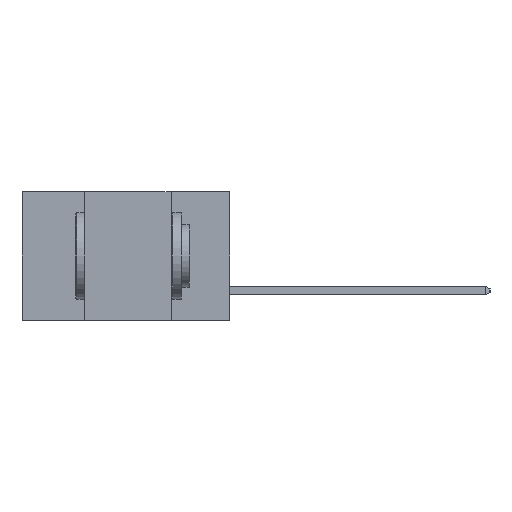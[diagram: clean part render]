
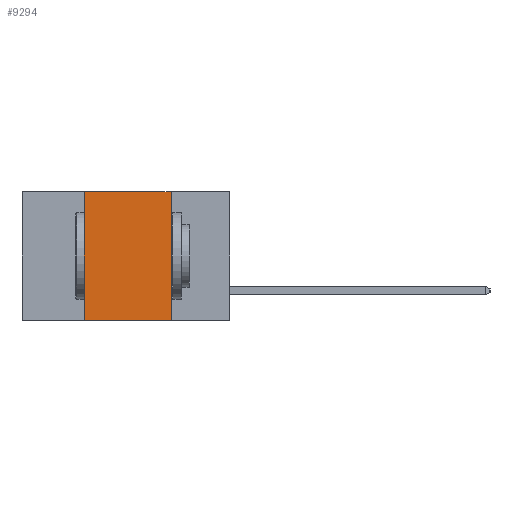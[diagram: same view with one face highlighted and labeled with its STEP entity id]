
A CAD part, left-side view. The second image highlights one B-rep face of the part: STEP entity #9294.
In plain terms, the highlighted planar face has unit normal (-1, 0, 0).
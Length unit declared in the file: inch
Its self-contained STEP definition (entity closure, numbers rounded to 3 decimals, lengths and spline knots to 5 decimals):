
#450 = ORIENTED_EDGE ( 'NONE', *, *, #6296, .F. ) ;
#673 = DIRECTION ( 'NONE',  ( 0., -1., 0. ) ) ;
#678 = LINE ( 'NONE', #5184, #2818 ) ;
#725 = DIRECTION ( 'NONE',  ( 0., -1., 0. ) ) ;
#744 = CARTESIAN_POINT ( 'NONE',  ( 0., 0.6, 0. ) ) ;
#784 = VECTOR ( 'NONE', #1436, 39.37008 ) ;
#842 = EDGE_CURVE ( 'NONE', #9845, #8155, #5381, .T. ) ;
#1018 = LINE ( 'NONE', #9768, #9151 ) ;
#1237 = EDGE_CURVE ( 'NONE', #9845, #6654, #1018, .T. ) ;
#1336 = ORIENTED_EDGE ( 'NONE', *, *, #1237, .T. ) ;
#1436 = DIRECTION ( 'NONE',  ( 0., 0., 1. ) ) ;
#1441 = CARTESIAN_POINT ( 'NONE',  ( 0., 0.42, -0.37 ) ) ;
#1471 = DIRECTION ( 'NONE',  ( 0., 0., -1. ) ) ;
#2467 = EDGE_CURVE ( 'NONE', #8155, #4888, #8090, .T. ) ;
#2547 = CARTESIAN_POINT ( 'NONE',  ( 0., 0.42, 0. ) ) ;
#2800 = CARTESIAN_POINT ( 'NONE',  ( 0., 0.17, -0.37 ) ) ;
#2818 = VECTOR ( 'NONE', #5220, 39.37008 ) ;
#2883 = ORIENTED_EDGE ( 'NONE', *, *, #2467, .F. ) ;
#2986 = ORIENTED_EDGE ( 'NONE', *, *, #842, .F. ) ;
#3768 = AXIS2_PLACEMENT_3D ( 'NONE', #5552, #6340, #1471 ) ;
#4430 = FACE_OUTER_BOUND ( 'NONE', #5604, .T. ) ;
#4532 = CARTESIAN_POINT ( 'NONE',  ( 0., 0.17, 0. ) ) ;
#4888 = VERTEX_POINT ( 'NONE', #4532 ) ;
#5184 = CARTESIAN_POINT ( 'NONE',  ( 0., 0.17, -0.37 ) ) ;
#5220 = DIRECTION ( 'NONE',  ( 0., 0., -1. ) ) ;
#5381 = LINE ( 'NONE', #1441, #784 ) ;
#5552 = CARTESIAN_POINT ( 'NONE',  ( 0., 0.6, 0. ) ) ;
#5604 = EDGE_LOOP ( 'NONE', ( #450, #2883, #2986, #1336 ) ) ;
#6234 = CARTESIAN_POINT ( 'NONE',  ( 0., 0.42, -0.37 ) ) ;
#6296 = EDGE_CURVE ( 'NONE', #4888, #6654, #678, .T. ) ;
#6340 = DIRECTION ( 'NONE',  ( 1., 0., 0. ) ) ;
#6654 = VERTEX_POINT ( 'NONE', #2800 ) ;
#8090 = LINE ( 'NONE', #744, #9759 ) ;
#8155 = VERTEX_POINT ( 'NONE', #2547 ) ;
#9151 = VECTOR ( 'NONE', #673, 39.37008 ) ;
#9294 = ADVANCED_FACE ( 'NONE', ( #4430 ), #9970, .F. ) ;
#9759 = VECTOR ( 'NONE', #725, 39.37008 ) ;
#9768 = CARTESIAN_POINT ( 'NONE',  ( 0., 0.6, -0.37 ) ) ;
#9845 = VERTEX_POINT ( 'NONE', #6234 ) ;
#9970 = PLANE ( 'NONE',  #3768 ) ;
